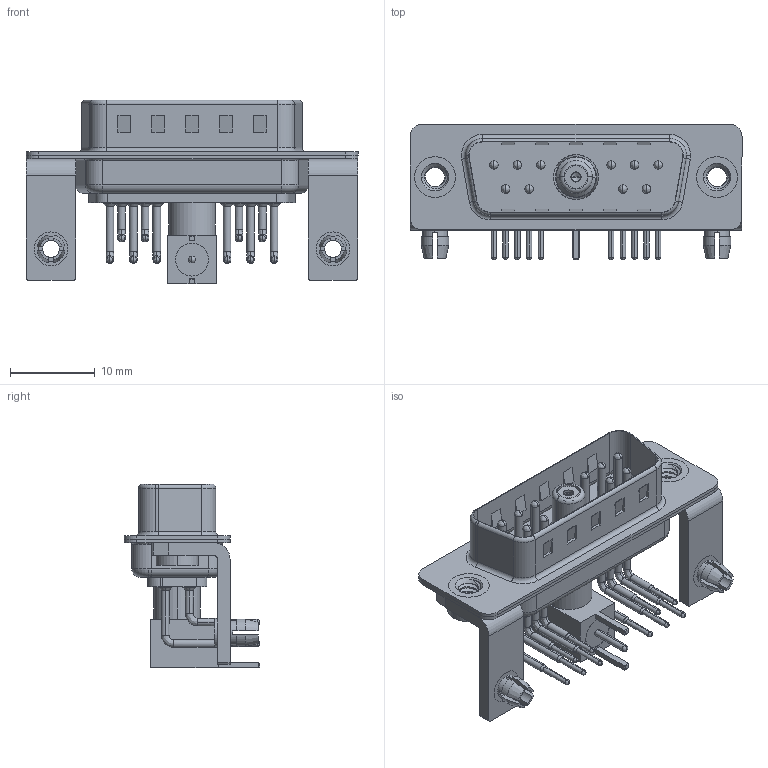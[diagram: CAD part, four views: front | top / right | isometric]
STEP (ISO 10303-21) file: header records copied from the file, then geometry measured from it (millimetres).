
FILE_DESCRIPTION (( 'STEP AP203' ), '1' );
FILE_NAME ('629-11W1240-7TB.STEP', '2022-05-06T22:05:21', ( '' ), ( '' ), 'SwSTEP 2.0', 'SolidWorks 2020', '' );
FILE_SCHEMA (( 'CONFIG_CONTROL_DESIGN' ));
Length unit declared in the file: millimetre
Products named in the file (17): Insulator Socket 2; 629Combo Board Lock; 629Combo Shell Rear_15 Contacts; 629Combo Stabilizer Bracket; Co-Ax Jack_RA PC Tail; Socket_RA; 629Combo Shell Front_15 Contacts; RA Back Shell; Co-Ax Jack Assy_RA; 629Combo Threaded Rivet_2; 629-11W1240-7TB; 629Combo Housing_11W1; 629Combo Contact Row 1; Insulator Socket; Locking Collar; Insulator RA Pin; 629Combo Contact Row 2
Assembly tree (27 placements, depth 3):
  629-11W1240-7TB
    629Combo Housing_11W1
    629Combo Shell Rear_15 Contacts
    629Combo Shell Front_15 Contacts
    629Combo Threaded Rivet_2  x2
    629Combo Stabilizer Bracket  x2
    629Combo Board Lock  x2
    Co-Ax Jack Assy_RA
      Co-Ax Jack_RA PC Tail
      Insulator Socket
      Insulator Socket 2
      Locking Collar
      Socket_RA
      RA Back Shell
      Insulator RA Pin
    629Combo Contact Row 1  x6
    629Combo Contact Row 2  x4
Bounding box: 39.2 x 16 x 21.71 mm (x, y, z)
Volume: 2559.6 mm3; surface area: 6930.6 mm2
Topology: 26 solids, 29 shells, 1745 faces, 4707 edges, 3041 vertices
Faces by surface type: plane 913, cylinder 620, cone 87, bspline 67, torus 56, sphere 2
Entity records: 28825 total; most frequent: CARTESIAN_POINT 6224, DIRECTION 4481, ORIENTED_EDGE 4148, EDGE_CURVE 2074, AXIS2_PLACEMENT_3D 1639, VERTEX_POINT 1335, LINE 1203, VECTOR 1203
